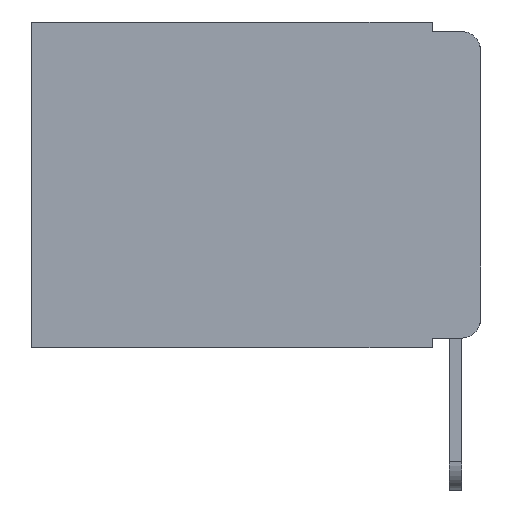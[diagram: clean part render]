
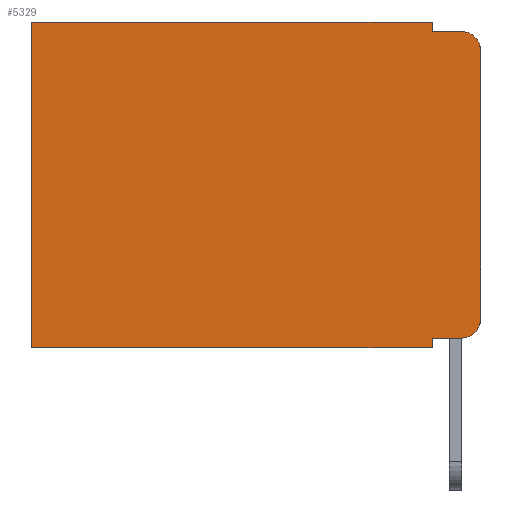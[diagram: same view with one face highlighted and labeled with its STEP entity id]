
A CAD part, left-side view. The second image highlights one B-rep face of the part: STEP entity #5329.
In plain terms, the highlighted planar face has unit normal (-1, 0, 0).
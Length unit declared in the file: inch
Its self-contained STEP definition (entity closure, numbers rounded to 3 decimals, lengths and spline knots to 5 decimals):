
#131 = CARTESIAN_POINT ( 'NONE',  ( 0.298, 0., 0. ) ) ;
#137 = CARTESIAN_POINT ( 'NONE',  ( 0.298, 0.473, -0.343 ) ) ;
#424 = VERTEX_POINT ( 'NONE', #11205 ) ;
#625 = EDGE_CURVE ( 'NONE', #8839, #2760, #1744, .T. ) ;
#631 = DIRECTION ( 'NONE',  ( 0., 0., -1. ) ) ;
#664 = EDGE_CURVE ( 'NONE', #3688, #9304, #3546, .T. ) ;
#879 = EDGE_CURVE ( 'NONE', #8364, #4840, #5324, .T. ) ;
#898 = EDGE_CURVE ( 'NONE', #8364, #8839, #9274, .T. ) ;
#925 = ORIENTED_EDGE ( 'NONE', *, *, #625, .T. ) ;
#1040 = ORIENTED_EDGE ( 'NONE', *, *, #2594, .F. ) ;
#1070 = EDGE_CURVE ( 'NONE', #424, #10304, #10891, .T. ) ;
#1266 = DIRECTION ( 'NONE',  ( 0., 0., -1. ) ) ;
#1319 = ORIENTED_EDGE ( 'NONE', *, *, #664, .F. ) ;
#1320 = CARTESIAN_POINT ( 'NONE',  ( 0.298, 0.051, -0.343 ) ) ;
#1411 = EDGE_LOOP ( 'NONE', ( #3891, #6172, #1040, #1319, #2937, #3464, #2140, #10314, #6688, #925 ) ) ;
#1530 = EDGE_CURVE ( 'NONE', #424, #2760, #5597, .T. ) ;
#1744 = CIRCLE ( 'NONE', #3436, 0.02 ) ;
#1793 = DIRECTION ( 'NONE',  ( 0., 1., 0. ) ) ;
#1804 = LINE ( 'NONE', #7560, #11350 ) ;
#1949 = EDGE_CURVE ( 'NONE', #8024, #5744, #2684, .T. ) ;
#1963 = PLANE ( 'NONE',  #10722 ) ;
#2140 = ORIENTED_EDGE ( 'NONE', *, *, #9769, .F. ) ;
#2594 = EDGE_CURVE ( 'NONE', #9304, #10304, #9073, .T. ) ;
#2684 = LINE ( 'NONE', #10169, #12029 ) ;
#2760 = VERTEX_POINT ( 'NONE', #11880 ) ;
#2937 = ORIENTED_EDGE ( 'NONE', *, *, #10156, .T. ) ;
#2968 = VECTOR ( 'NONE', #10638, 39.37008 ) ;
#3018 = VECTOR ( 'NONE', #8273, 39.37008 ) ;
#3028 = CARTESIAN_POINT ( 'NONE',  ( 0.298, 0., 0. ) ) ;
#3309 = CARTESIAN_POINT ( 'NONE',  ( 0.298, 0.051, -0.333 ) ) ;
#3397 = CARTESIAN_POINT ( 'NONE',  ( 0.298, 0.02, -0.313 ) ) ;
#3436 = AXIS2_PLACEMENT_3D ( 'NONE', #3397, #9694, #9931 ) ;
#3464 = ORIENTED_EDGE ( 'NONE', *, *, #1949, .T. ) ;
#3546 = LINE ( 'NONE', #4182, #5780 ) ;
#3688 = VERTEX_POINT ( 'NONE', #10394 ) ;
#3891 = ORIENTED_EDGE ( 'NONE', *, *, #1530, .F. ) ;
#4043 = DIRECTION ( 'NONE',  ( 0., 0., -1. ) ) ;
#4182 = CARTESIAN_POINT ( 'NONE',  ( 0.298, 0.051, 0. ) ) ;
#4596 = FACE_OUTER_BOUND ( 'NONE', #1411, .T. ) ;
#4840 = VERTEX_POINT ( 'NONE', #1320 ) ;
#5037 = VECTOR ( 'NONE', #11558, 39.37008 ) ;
#5324 = LINE ( 'NONE', #7428, #5037 ) ;
#5329 = ADVANCED_FACE ( 'NONE', ( #4596 ), #1963, .F. ) ;
#5521 = AXIS2_PLACEMENT_3D ( 'NONE', #11414, #11389, #631 ) ;
#5546 = LINE ( 'NONE', #9764, #2968 ) ;
#5597 = LINE ( 'NONE', #131, #3018 ) ;
#5744 = VERTEX_POINT ( 'NONE', #137 ) ;
#5780 = VECTOR ( 'NONE', #1266, 39.37008 ) ;
#5861 = VECTOR ( 'NONE', #11245, 39.37008 ) ;
#6172 = ORIENTED_EDGE ( 'NONE', *, *, #1070, .T. ) ;
#6688 = ORIENTED_EDGE ( 'NONE', *, *, #898, .T. ) ;
#7214 = CARTESIAN_POINT ( 'NONE',  ( 0.298, 0.051, -0.333 ) ) ;
#7315 = DIRECTION ( 'NONE',  ( 0., -1., 0. ) ) ;
#7428 = CARTESIAN_POINT ( 'NONE',  ( 0.298, 0.051, 0. ) ) ;
#7560 = CARTESIAN_POINT ( 'NONE',  ( 0.298, 0., 0. ) ) ;
#8024 = VERTEX_POINT ( 'NONE', #10198 ) ;
#8271 = CARTESIAN_POINT ( 'NONE',  ( 0.298, 0.051, -0.01 ) ) ;
#8273 = DIRECTION ( 'NONE',  ( 0., 0., -1. ) ) ;
#8364 = VERTEX_POINT ( 'NONE', #3309 ) ;
#8741 = DIRECTION ( 'NONE',  ( 0., 0., -1. ) ) ;
#8839 = VERTEX_POINT ( 'NONE', #9466 ) ;
#9073 = LINE ( 'NONE', #11197, #5861 ) ;
#9274 = LINE ( 'NONE', #7214, #11569 ) ;
#9304 = VERTEX_POINT ( 'NONE', #8271 ) ;
#9466 = CARTESIAN_POINT ( 'NONE',  ( 0.298, 0.02, -0.333 ) ) ;
#9477 = CARTESIAN_POINT ( 'NONE',  ( 0.298, 0.02, -0.01 ) ) ;
#9519 = DIRECTION ( 'NONE',  ( 1., 0., 0. ) ) ;
#9694 = DIRECTION ( 'NONE',  ( -1., 0., 0. ) ) ;
#9764 = CARTESIAN_POINT ( 'NONE',  ( 0.298, 0., -0.343 ) ) ;
#9769 = EDGE_CURVE ( 'NONE', #4840, #5744, #5546, .T. ) ;
#9931 = DIRECTION ( 'NONE',  ( 0., 0., -1. ) ) ;
#10156 = EDGE_CURVE ( 'NONE', #3688, #8024, #1804, .T. ) ;
#10169 = CARTESIAN_POINT ( 'NONE',  ( 0.298, 0.473, 0. ) ) ;
#10198 = CARTESIAN_POINT ( 'NONE',  ( 0.298, 0.473, 0. ) ) ;
#10304 = VERTEX_POINT ( 'NONE', #9477 ) ;
#10314 = ORIENTED_EDGE ( 'NONE', *, *, #879, .F. ) ;
#10394 = CARTESIAN_POINT ( 'NONE',  ( 0.298, 0.051, 0. ) ) ;
#10638 = DIRECTION ( 'NONE',  ( 0., 1., 0. ) ) ;
#10722 = AXIS2_PLACEMENT_3D ( 'NONE', #3028, #9519, #4043 ) ;
#10891 = CIRCLE ( 'NONE', #5521, 0.02 ) ;
#11197 = CARTESIAN_POINT ( 'NONE',  ( 0.298, 0.051, -0.01 ) ) ;
#11205 = CARTESIAN_POINT ( 'NONE',  ( 0.298, 0., -0.03 ) ) ;
#11245 = DIRECTION ( 'NONE',  ( 0., -1., 0. ) ) ;
#11350 = VECTOR ( 'NONE', #1793, 39.37008 ) ;
#11389 = DIRECTION ( 'NONE',  ( -1., 0., 0. ) ) ;
#11414 = CARTESIAN_POINT ( 'NONE',  ( 0.298, 0.02, -0.03 ) ) ;
#11558 = DIRECTION ( 'NONE',  ( 0., 0., -1. ) ) ;
#11569 = VECTOR ( 'NONE', #7315, 39.37008 ) ;
#11880 = CARTESIAN_POINT ( 'NONE',  ( 0.298, 0., -0.313 ) ) ;
#12029 = VECTOR ( 'NONE', #8741, 39.37008 ) ;
